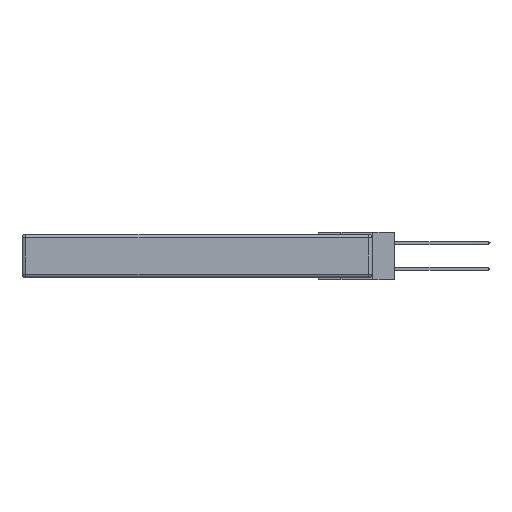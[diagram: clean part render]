
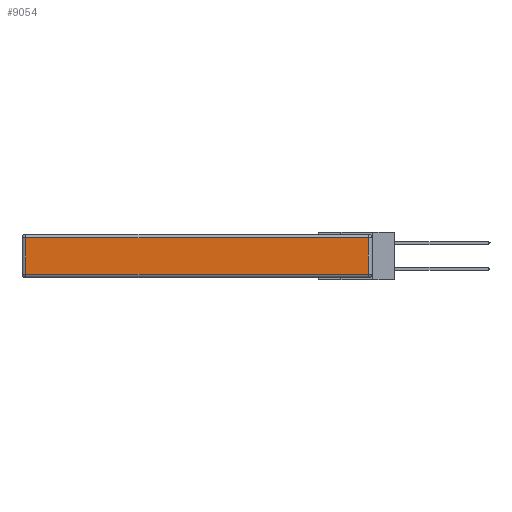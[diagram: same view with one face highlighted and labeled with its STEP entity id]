
A CAD part, left-side view. The second image highlights one B-rep face of the part: STEP entity #9054.
In plain terms, the highlighted planar face has unit normal (-1, 0, 0).
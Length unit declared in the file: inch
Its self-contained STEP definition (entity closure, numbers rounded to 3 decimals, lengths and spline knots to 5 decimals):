
#304 = ORIENTED_EDGE ( 'NONE', *, *, #8828, .T. ) ;
#688 = DIRECTION ( 'NONE',  ( -1., 0., 0. ) ) ;
#1337 = EDGE_CURVE ( 'NONE', #9438, #14114, #1376, .T. ) ;
#1376 = LINE ( 'NONE', #8347, #16115 ) ;
#1990 = DIRECTION ( 'NONE',  ( 0., 0., 1. ) ) ;
#2275 = VERTEX_POINT ( 'NONE', #10580 ) ;
#2827 = ORIENTED_EDGE ( 'NONE', *, *, #14984, .T. ) ;
#2980 = DIRECTION ( 'NONE',  ( 0., 0., 1. ) ) ;
#3590 = LINE ( 'NONE', #15906, #10368 ) ;
#4694 = CARTESIAN_POINT ( 'NONE',  ( 0., 0.03, -0.03 ) ) ;
#5171 = CARTESIAN_POINT ( 'NONE',  ( 0., 2.75, -0.03 ) ) ;
#6008 = CARTESIAN_POINT ( 'NONE',  ( 0., 0.03, -0.313 ) ) ;
#6012 = PLANE ( 'NONE',  #11073 ) ;
#6943 = LINE ( 'NONE', #5171, #9274 ) ;
#7015 = CARTESIAN_POINT ( 'NONE',  ( 0., 2.72, -0.03 ) ) ;
#8347 = CARTESIAN_POINT ( 'NONE',  ( 0., 0.03, -0.343 ) ) ;
#8828 = EDGE_CURVE ( 'NONE', #13231, #2275, #3590, .T. ) ;
#9054 = ADVANCED_FACE ( 'NONE', ( #17298 ), #6012, .T. ) ;
#9274 = VECTOR ( 'NONE', #15840, 39.37008 ) ;
#9438 = VERTEX_POINT ( 'NONE', #6008 ) ;
#10368 = VECTOR ( 'NONE', #12075, 39.37008 ) ;
#10580 = CARTESIAN_POINT ( 'NONE',  ( 0., 2.72, -0.313 ) ) ;
#10851 = EDGE_CURVE ( 'NONE', #14114, #13231, #6943, .T. ) ;
#11073 = AXIS2_PLACEMENT_3D ( 'NONE', #15426, #688, #1990 ) ;
#11472 = ORIENTED_EDGE ( 'NONE', *, *, #10851, .T. ) ;
#11513 = LINE ( 'NONE', #14717, #12577 ) ;
#11978 = DIRECTION ( 'NONE',  ( 0., -1., 0. ) ) ;
#12075 = DIRECTION ( 'NONE',  ( 0., 0., -1. ) ) ;
#12577 = VECTOR ( 'NONE', #11978, 39.37008 ) ;
#13231 = VERTEX_POINT ( 'NONE', #7015 ) ;
#14114 = VERTEX_POINT ( 'NONE', #4694 ) ;
#14717 = CARTESIAN_POINT ( 'NONE',  ( 0., 0., -0.313 ) ) ;
#14984 = EDGE_CURVE ( 'NONE', #2275, #9438, #11513, .T. ) ;
#15426 = CARTESIAN_POINT ( 'NONE',  ( 0., 0., -0.343 ) ) ;
#15840 = DIRECTION ( 'NONE',  ( 0., 1., 0. ) ) ;
#15906 = CARTESIAN_POINT ( 'NONE',  ( 0., 2.72, -0.343 ) ) ;
#16115 = VECTOR ( 'NONE', #2980, 39.37008 ) ;
#16524 = EDGE_LOOP ( 'NONE', ( #2827, #17379, #11472, #304 ) ) ;
#17298 = FACE_OUTER_BOUND ( 'NONE', #16524, .T. ) ;
#17379 = ORIENTED_EDGE ( 'NONE', *, *, #1337, .T. ) ;
